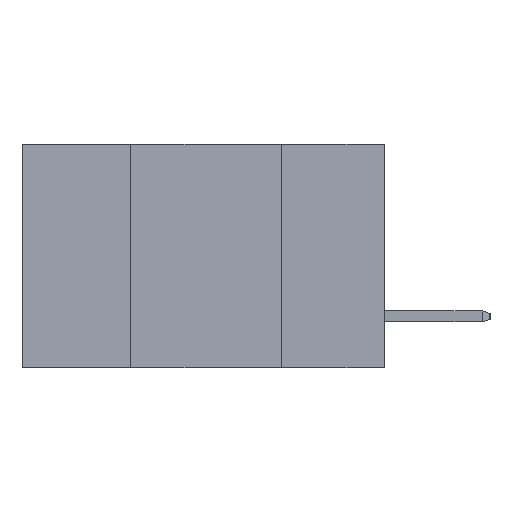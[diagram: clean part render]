
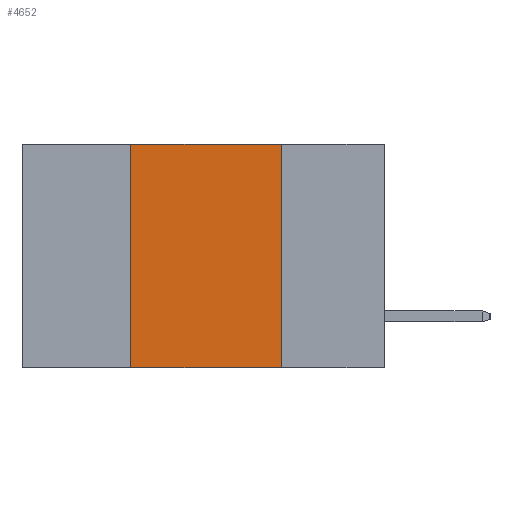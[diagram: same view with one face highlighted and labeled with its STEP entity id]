
A CAD part, left-side view. The second image highlights one B-rep face of the part: STEP entity #4652.
In plain terms, the highlighted planar face has unit normal (-1, 0, 0).
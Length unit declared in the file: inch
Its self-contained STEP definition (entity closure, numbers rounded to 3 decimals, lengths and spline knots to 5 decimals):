
#2 = VECTOR ( 'NONE', #6140, 39.37008 ) ;
#574 = DIRECTION ( 'NONE',  ( 1., 0., 0. ) ) ;
#4300 = LINE ( 'NONE', #4787, #17395 ) ;
#4612 = CARTESIAN_POINT ( 'NONE',  ( 0., 0.42, 0. ) ) ;
#4652 = ADVANCED_FACE ( 'NONE', ( #14185 ), #10925, .F. ) ;
#4787 = CARTESIAN_POINT ( 'NONE',  ( 0., 0.6, 0. ) ) ;
#4836 = CARTESIAN_POINT ( 'NONE',  ( 0., 0.17, 0. ) ) ;
#5387 = VECTOR ( 'NONE', #18351, 39.37008 ) ;
#5709 = LINE ( 'NONE', #21406, #2 ) ;
#5903 = VERTEX_POINT ( 'NONE', #21083 ) ;
#6140 = DIRECTION ( 'NONE',  ( 0., 0., -1. ) ) ;
#6492 = EDGE_CURVE ( 'NONE', #5903, #13551, #6541, .T. ) ;
#6541 = LINE ( 'NONE', #10051, #11158 ) ;
#7442 = CARTESIAN_POINT ( 'NONE',  ( 0., 0.6, 0. ) ) ;
#7659 = EDGE_CURVE ( 'NONE', #15633, #8138, #5709, .T. ) ;
#8138 = VERTEX_POINT ( 'NONE', #10880 ) ;
#9632 = ORIENTED_EDGE ( 'NONE', *, *, #21808, .F. ) ;
#10051 = CARTESIAN_POINT ( 'NONE',  ( 0., 0.42, 0. ) ) ;
#10880 = CARTESIAN_POINT ( 'NONE',  ( 0., 0.17, -0.37 ) ) ;
#10925 = PLANE ( 'NONE',  #21072 ) ;
#11158 = VECTOR ( 'NONE', #20187, 39.37008 ) ;
#12182 = EDGE_LOOP ( 'NONE', ( #13001, #9632, #14759, #18811 ) ) ;
#12644 = DIRECTION ( 'NONE',  ( 0., 0., -1. ) ) ;
#13001 = ORIENTED_EDGE ( 'NONE', *, *, #7659, .F. ) ;
#13436 = DIRECTION ( 'NONE',  ( 0., -1., 0. ) ) ;
#13551 = VERTEX_POINT ( 'NONE', #4612 ) ;
#14185 = FACE_OUTER_BOUND ( 'NONE', #12182, .T. ) ;
#14759 = ORIENTED_EDGE ( 'NONE', *, *, #6492, .F. ) ;
#15012 = CARTESIAN_POINT ( 'NONE',  ( 0., 0.6, -0.37 ) ) ;
#15633 = VERTEX_POINT ( 'NONE', #4836 ) ;
#17395 = VECTOR ( 'NONE', #13436, 39.37008 ) ;
#18351 = DIRECTION ( 'NONE',  ( 0., -1., 0. ) ) ;
#18452 = LINE ( 'NONE', #15012, #5387 ) ;
#18811 = ORIENTED_EDGE ( 'NONE', *, *, #21778, .T. ) ;
#20187 = DIRECTION ( 'NONE',  ( 0., 0., 1. ) ) ;
#21072 = AXIS2_PLACEMENT_3D ( 'NONE', #7442, #574, #12644 ) ;
#21083 = CARTESIAN_POINT ( 'NONE',  ( 0., 0.42, -0.37 ) ) ;
#21406 = CARTESIAN_POINT ( 'NONE',  ( 0., 0.17, 0. ) ) ;
#21778 = EDGE_CURVE ( 'NONE', #5903, #8138, #18452, .T. ) ;
#21808 = EDGE_CURVE ( 'NONE', #13551, #15633, #4300, .T. ) ;
